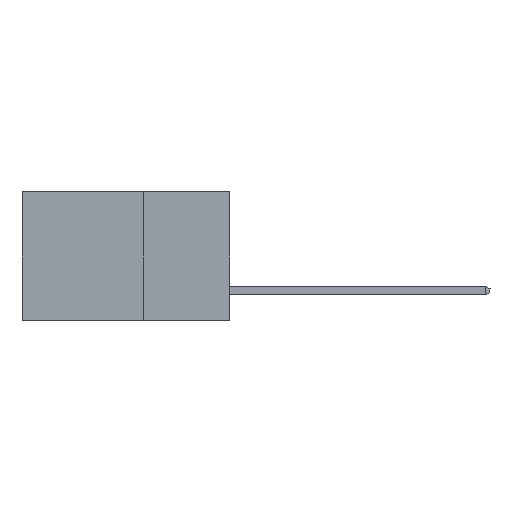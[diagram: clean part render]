
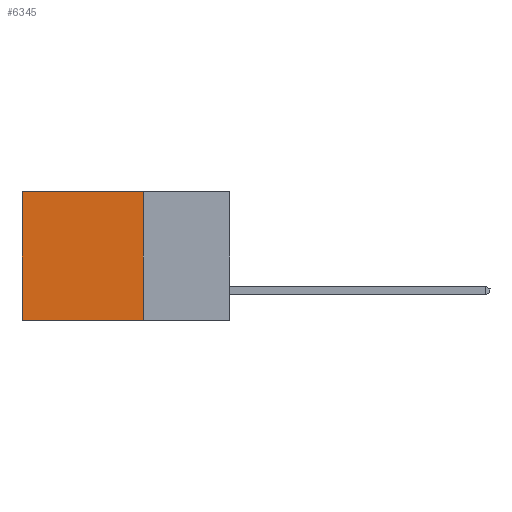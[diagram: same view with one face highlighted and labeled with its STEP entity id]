
A CAD part, left-side view. The second image highlights one B-rep face of the part: STEP entity #6345.
In plain terms, the highlighted planar face has unit normal (-1, 0, 0).
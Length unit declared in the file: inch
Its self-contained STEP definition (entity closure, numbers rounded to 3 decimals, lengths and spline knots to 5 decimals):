
#55 = AXIS2_PLACEMENT_3D ( 'NONE', #15653, #8070, #13776 ) ;
#270 = CARTESIAN_POINT ( 'NONE',  ( 0.2615, 0.6, -0.37 ) ) ;
#375 = CARTESIAN_POINT ( 'NONE',  ( 0.2615, 0.25, 0. ) ) ;
#385 = VERTEX_POINT ( 'NONE', #6427 ) ;
#1284 = DIRECTION ( 'NONE',  ( 0., 0., -1. ) ) ;
#1350 = FACE_OUTER_BOUND ( 'NONE', #11346, .T. ) ;
#3127 = EDGE_CURVE ( 'NONE', #385, #12689, #10117, .T. ) ;
#4435 = VECTOR ( 'NONE', #9981, 39.37008 ) ;
#4682 = EDGE_CURVE ( 'NONE', #385, #9858, #14506, .T. ) ;
#6345 = ADVANCED_FACE ( 'NONE', ( #1350 ), #18169, .F. ) ;
#6427 = CARTESIAN_POINT ( 'NONE',  ( 0.2615, 0.25, 0. ) ) ;
#7081 = LINE ( 'NONE', #12797, #4435 ) ;
#7799 = VECTOR ( 'NONE', #13479, 39.37008 ) ;
#8070 = DIRECTION ( 'NONE',  ( 1., 0., 0. ) ) ;
#8976 = CARTESIAN_POINT ( 'NONE',  ( 0.2615, 0.25, -0.37 ) ) ;
#9423 = VECTOR ( 'NONE', #1284, 39.37008 ) ;
#9832 = ORIENTED_EDGE ( 'NONE', *, *, #15712, .T. ) ;
#9858 = VERTEX_POINT ( 'NONE', #14577 ) ;
#9981 = DIRECTION ( 'NONE',  ( 0., 1., 0. ) ) ;
#10117 = LINE ( 'NONE', #375, #16711 ) ;
#10372 = EDGE_CURVE ( 'NONE', #9858, #17028, #7081, .T. ) ;
#10778 = CARTESIAN_POINT ( 'NONE',  ( 0.2615, 0.6, 0. ) ) ;
#11346 = EDGE_LOOP ( 'NONE', ( #9832, #14864, #18107, #14922 ) ) ;
#12689 = VERTEX_POINT ( 'NONE', #10778 ) ;
#12797 = CARTESIAN_POINT ( 'NONE',  ( 0.2615, 0.25, -0.37 ) ) ;
#13479 = DIRECTION ( 'NONE',  ( 0., 0., -1. ) ) ;
#13776 = DIRECTION ( 'NONE',  ( 0., 0., -1. ) ) ;
#14081 = LINE ( 'NONE', #18480, #9423 ) ;
#14506 = LINE ( 'NONE', #8976, #7799 ) ;
#14577 = CARTESIAN_POINT ( 'NONE',  ( 0.2615, 0.25, -0.37 ) ) ;
#14864 = ORIENTED_EDGE ( 'NONE', *, *, #10372, .F. ) ;
#14922 = ORIENTED_EDGE ( 'NONE', *, *, #3127, .T. ) ;
#15653 = CARTESIAN_POINT ( 'NONE',  ( 0.2615, 0.25, -0.37 ) ) ;
#15712 = EDGE_CURVE ( 'NONE', #12689, #17028, #14081, .T. ) ;
#15744 = DIRECTION ( 'NONE',  ( 0., 1., 0. ) ) ;
#16711 = VECTOR ( 'NONE', #15744, 39.37008 ) ;
#17028 = VERTEX_POINT ( 'NONE', #270 ) ;
#18107 = ORIENTED_EDGE ( 'NONE', *, *, #4682, .F. ) ;
#18169 = PLANE ( 'NONE',  #55 ) ;
#18480 = CARTESIAN_POINT ( 'NONE',  ( 0.2615, 0.6, -0.37 ) ) ;
